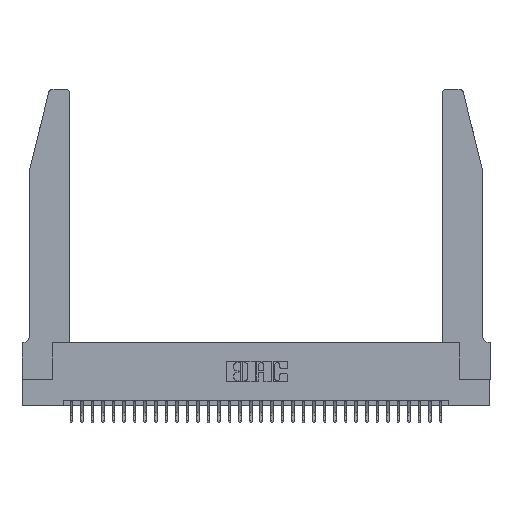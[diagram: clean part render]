
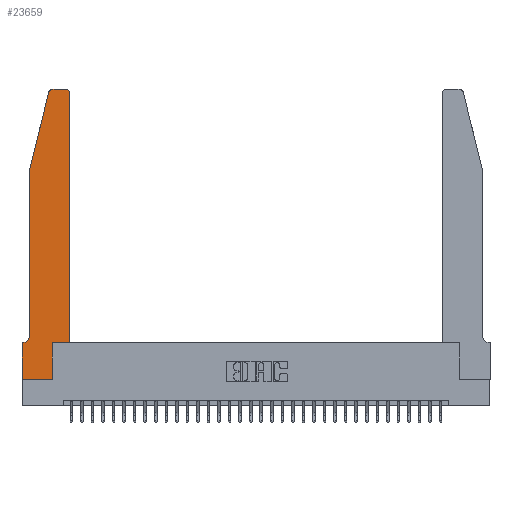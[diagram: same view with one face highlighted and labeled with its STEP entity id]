
A CAD part, top view. The second image highlights one B-rep face of the part: STEP entity #23659.
In plain terms, the highlighted planar face has unit normal (0, 0, 1).
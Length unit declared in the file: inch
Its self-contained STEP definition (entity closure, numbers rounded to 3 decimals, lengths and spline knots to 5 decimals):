
#156 = CARTESIAN_POINT ( 'NONE',  ( 0.0755, 2., 0.37 ) ) ;
#955 = EDGE_CURVE ( 'NONE', #24571, #10615, #25392, .T. ) ;
#1025 = LINE ( 'NONE', #30214, #7267 ) ;
#1398 = VECTOR ( 'NONE', #28766, 39.37008 ) ;
#1628 = DIRECTION ( 'NONE',  ( 1., 0., 0. ) ) ;
#2653 = EDGE_CURVE ( 'NONE', #13002, #11309, #30632, .T. ) ;
#2991 = CARTESIAN_POINT ( 'NONE',  ( 0.0055, 0.35, 0.37 ) ) ;
#3551 = CARTESIAN_POINT ( 'NONE',  ( 0.0755, 0.42, 0.37 ) ) ;
#4325 = LINE ( 'NONE', #18430, #17585 ) ;
#5286 = DIRECTION ( 'NONE',  ( 1., 0., 0. ) ) ;
#5506 = VERTEX_POINT ( 'NONE', #3551 ) ;
#5650 = EDGE_CURVE ( 'NONE', #31334, #24203, #20274, .T. ) ;
#6244 = VERTEX_POINT ( 'NONE', #22296 ) ;
#6582 = FACE_OUTER_BOUND ( 'NONE', #17091, .T. ) ;
#6900 = CARTESIAN_POINT ( 'NONE',  ( 0.25487, 2.72718, 0.37 ) ) ;
#6988 = EDGE_CURVE ( 'NONE', #13588, #31423, #29565, .T. ) ;
#7267 = VECTOR ( 'NONE', #32835, 39.37008 ) ;
#7809 = VERTEX_POINT ( 'NONE', #18676 ) ;
#8005 = ORIENTED_EDGE ( 'NONE', *, *, #27867, .T. ) ;
#8534 = ORIENTED_EDGE ( 'NONE', *, *, #14146, .T. ) ;
#8649 = AXIS2_PLACEMENT_3D ( 'NONE', #17674, #17569, #15005 ) ;
#8770 = ORIENTED_EDGE ( 'NONE', *, *, #25864, .T. ) ;
#9046 = ORIENTED_EDGE ( 'NONE', *, *, #25467, .T. ) ;
#9274 = ORIENTED_EDGE ( 'NONE', *, *, #2653, .T. ) ;
#9307 = CARTESIAN_POINT ( 'NONE',  ( 0., 0., 0.37 ) ) ;
#9315 = CARTESIAN_POINT ( 'NONE',  ( 0.0055, 0.42, 0.37 ) ) ;
#9551 = ORIENTED_EDGE ( 'NONE', *, *, #5650, .T. ) ;
#9681 = ORIENTED_EDGE ( 'NONE', *, *, #15915, .T. ) ;
#9706 = ORIENTED_EDGE ( 'NONE', *, *, #23786, .T. ) ;
#9976 = ORIENTED_EDGE ( 'NONE', *, *, #14963, .T. ) ;
#10006 = EDGE_CURVE ( 'NONE', #31423, #24571, #22813, .T. ) ;
#10013 = ORIENTED_EDGE ( 'NONE', *, *, #955, .T. ) ;
#10487 = DIRECTION ( 'NONE',  ( 0., 0., 1. ) ) ;
#10615 = VERTEX_POINT ( 'NONE', #6900 ) ;
#10783 = CARTESIAN_POINT ( 'NONE',  ( 0.4505, 0.35, 0.37 ) ) ;
#10803 = ORIENTED_EDGE ( 'NONE', *, *, #6988, .T. ) ;
#11009 = AXIS2_PLACEMENT_3D ( 'NONE', #33077, #17504, #1628 ) ;
#11078 = CARTESIAN_POINT ( 'NONE',  ( 0.2865, 0., 0.37 ) ) ;
#11309 = VERTEX_POINT ( 'NONE', #11078 ) ;
#12019 = DIRECTION ( 'NONE',  ( -1., 0., 0. ) ) ;
#12695 = DIRECTION ( 'NONE',  ( -1., 0., 0. ) ) ;
#13002 = VERTEX_POINT ( 'NONE', #15331 ) ;
#13588 = VERTEX_POINT ( 'NONE', #26289 ) ;
#14146 = EDGE_CURVE ( 'NONE', #30775, #13588, #27790, .T. ) ;
#14602 = AXIS2_PLACEMENT_3D ( 'NONE', #9315, #27577, #12019 ) ;
#14963 = EDGE_CURVE ( 'NONE', #24203, #13002, #15543, .T. ) ;
#15005 = DIRECTION ( 'NONE',  ( 1., 0., 0. ) ) ;
#15062 = CARTESIAN_POINT ( 'NONE',  ( 0., 0.35, 0.37 ) ) ;
#15331 = CARTESIAN_POINT ( 'NONE',  ( 0., 0., 0.37 ) ) ;
#15543 = LINE ( 'NONE', #20902, #1398 ) ;
#15851 = VECTOR ( 'NONE', #17372, 39.37008 ) ;
#15915 = EDGE_CURVE ( 'NONE', #5506, #31334, #22349, .T. ) ;
#17091 = EDGE_LOOP ( 'NONE', ( #31721, #10013, #8005, #9706, #9681, #9551, #9976, #9274, #9046, #8770, #8534, #10803 ) ) ;
#17372 = DIRECTION ( 'NONE',  ( -1., 0., 0. ) ) ;
#17504 = DIRECTION ( 'NONE',  ( 0., 0., 1. ) ) ;
#17569 = DIRECTION ( 'NONE',  ( 0., 0., 1. ) ) ;
#17585 = VECTOR ( 'NONE', #5286, 39.37008 ) ;
#17674 = CARTESIAN_POINT ( 'NONE',  ( 0.284, 2.72, 0.37 ) ) ;
#17827 = VECTOR ( 'NONE', #21941, 39.37008 ) ;
#18430 = CARTESIAN_POINT ( 'NONE',  ( 0.4505, 0.35, 0.37 ) ) ;
#18676 = CARTESIAN_POINT ( 'NONE',  ( 0.0755, 2., 0.37 ) ) ;
#19329 = CARTESIAN_POINT ( 'NONE',  ( 0.0755, 2., 0.37 ) ) ;
#20274 = LINE ( 'NONE', #30335, #15851 ) ;
#20735 = CARTESIAN_POINT ( 'NONE',  ( 0., 0.35, 0.37 ) ) ;
#20902 = CARTESIAN_POINT ( 'NONE',  ( 0., 0., 0.37 ) ) ;
#21472 = CARTESIAN_POINT ( 'NONE',  ( 0.284, 2.75, 0.37 ) ) ;
#21941 = DIRECTION ( 'NONE',  ( -0.239, -0.971, 0. ) ) ;
#22296 = CARTESIAN_POINT ( 'NONE',  ( 0.2865, 0.35, 0.37 ) ) ;
#22349 = CIRCLE ( 'NONE', #14602, 0.07 ) ;
#22813 = LINE ( 'NONE', #25646, #29766 ) ;
#23659 = ADVANCED_FACE ( 'NONE', ( #6582 ), #26099, .T. ) ;
#23678 = VECTOR ( 'NONE', #24956, 39.37008 ) ;
#23786 = EDGE_CURVE ( 'NONE', #7809, #5506, #31999, .T. ) ;
#23915 = DIRECTION ( 'NONE',  ( 0., -1., 0. ) ) ;
#24203 = VERTEX_POINT ( 'NONE', #15062 ) ;
#24571 = VERTEX_POINT ( 'NONE', #21472 ) ;
#24956 = DIRECTION ( 'NONE',  ( 1., 0., 0. ) ) ;
#25304 = CARTESIAN_POINT ( 'NONE',  ( 0.4505, 0.35, 0.37 ) ) ;
#25392 = CIRCLE ( 'NONE', #8649, 0.03 ) ;
#25467 = EDGE_CURVE ( 'NONE', #11309, #6244, #1025, .T. ) ;
#25646 = CARTESIAN_POINT ( 'NONE',  ( 0.2605, 2.75, 0.37 ) ) ;
#25802 = AXIS2_PLACEMENT_3D ( 'NONE', #20735, #10487, #28701 ) ;
#25864 = EDGE_CURVE ( 'NONE', #6244, #30775, #4325, .T. ) ;
#26099 = PLANE ( 'NONE',  #25802 ) ;
#26289 = CARTESIAN_POINT ( 'NONE',  ( 0.4505, 2.72, 0.37 ) ) ;
#27018 = CARTESIAN_POINT ( 'NONE',  ( 0.4205, 2.75, 0.37 ) ) ;
#27577 = DIRECTION ( 'NONE',  ( 0., 0., -1. ) ) ;
#27790 = LINE ( 'NONE', #25304, #33886 ) ;
#27867 = EDGE_CURVE ( 'NONE', #10615, #7809, #31703, .T. ) ;
#28017 = DIRECTION ( 'NONE',  ( 0., 1., 0. ) ) ;
#28701 = DIRECTION ( 'NONE',  ( 1., 0., 0. ) ) ;
#28766 = DIRECTION ( 'NONE',  ( 0., -1., 0. ) ) ;
#29565 = CIRCLE ( 'NONE', #11009, 0.03 ) ;
#29766 = VECTOR ( 'NONE', #12695, 39.37008 ) ;
#30214 = CARTESIAN_POINT ( 'NONE',  ( 0.2865, 0.35, 0.37 ) ) ;
#30335 = CARTESIAN_POINT ( 'NONE',  ( 0.0755, 0.35, 0.37 ) ) ;
#30356 = VECTOR ( 'NONE', #23915, 39.37008 ) ;
#30632 = LINE ( 'NONE', #9307, #23678 ) ;
#30775 = VERTEX_POINT ( 'NONE', #10783 ) ;
#31334 = VERTEX_POINT ( 'NONE', #2991 ) ;
#31423 = VERTEX_POINT ( 'NONE', #27018 ) ;
#31703 = LINE ( 'NONE', #19329, #17827 ) ;
#31721 = ORIENTED_EDGE ( 'NONE', *, *, #10006, .T. ) ;
#31999 = LINE ( 'NONE', #156, #30356 ) ;
#32835 = DIRECTION ( 'NONE',  ( 0., 1., 0. ) ) ;
#33077 = CARTESIAN_POINT ( 'NONE',  ( 0.4205, 2.72, 0.37 ) ) ;
#33886 = VECTOR ( 'NONE', #28017, 39.37008 ) ;
